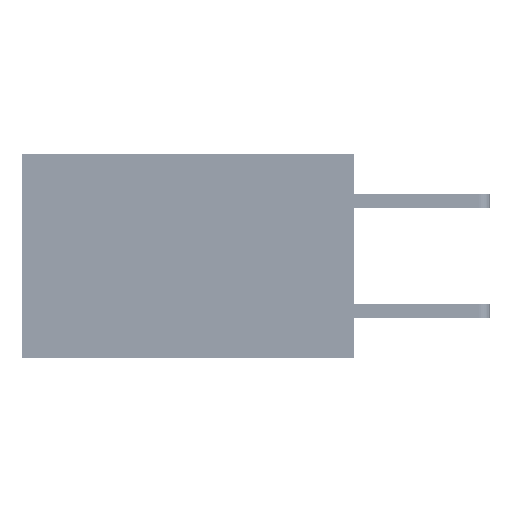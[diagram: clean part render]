
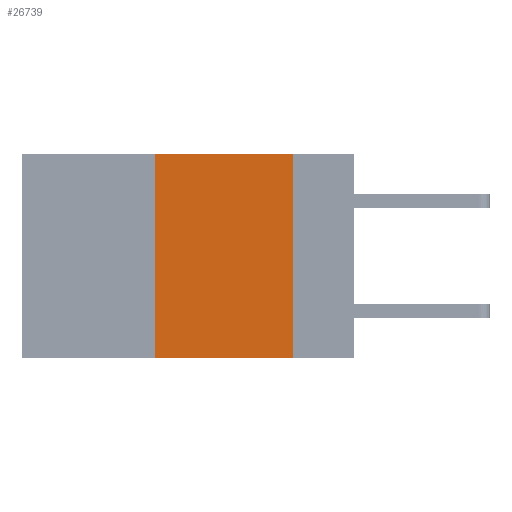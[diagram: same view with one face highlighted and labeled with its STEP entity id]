
A CAD part, left-side view. The second image highlights one B-rep face of the part: STEP entity #26739.
In plain terms, the highlighted planar face has unit normal (-1, 0, 0).
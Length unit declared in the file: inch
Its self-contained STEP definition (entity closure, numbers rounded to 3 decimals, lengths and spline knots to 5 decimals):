
#411 = VECTOR ( 'NONE', #22511, 39.37008 ) ;
#1099 = LINE ( 'NONE', #14853, #40923 ) ;
#1302 = CARTESIAN_POINT ( 'NONE',  ( 0., 0.11, 0. ) ) ;
#3840 = DIRECTION ( 'NONE',  ( 0., -1., 0. ) ) ;
#5320 = CARTESIAN_POINT ( 'NONE',  ( 0., 0.6, 0. ) ) ;
#7498 = CARTESIAN_POINT ( 'NONE',  ( 0., 0.6, 0. ) ) ;
#9156 = CARTESIAN_POINT ( 'NONE',  ( 0., 0.11, 0. ) ) ;
#10337 = VECTOR ( 'NONE', #22855, 39.37008 ) ;
#11505 = VECTOR ( 'NONE', #3840, 39.37008 ) ;
#14853 = CARTESIAN_POINT ( 'NONE',  ( 0., 0.6, -0.37 ) ) ;
#15875 = VERTEX_POINT ( 'NONE', #21773 ) ;
#17239 = AXIS2_PLACEMENT_3D ( 'NONE', #5320, #35069, #21687 ) ;
#17415 = CARTESIAN_POINT ( 'NONE',  ( 0., 0.36, 0. ) ) ;
#18458 = PLANE ( 'NONE',  #17239 ) ;
#20668 = EDGE_CURVE ( 'NONE', #32544, #28873, #37036, .T. ) ;
#20706 = CARTESIAN_POINT ( 'NONE',  ( 0., 0.11, -0.37 ) ) ;
#21687 = DIRECTION ( 'NONE',  ( 0., 0., -1. ) ) ;
#21773 = CARTESIAN_POINT ( 'NONE',  ( 0., 0.36, -0.37 ) ) ;
#22511 = DIRECTION ( 'NONE',  ( 0., 0., -1. ) ) ;
#22855 = DIRECTION ( 'NONE',  ( 0., 0., 1. ) ) ;
#25142 = FACE_OUTER_BOUND ( 'NONE', #33915, .T. ) ;
#26739 = ADVANCED_FACE ( 'NONE', ( #25142 ), #18458, .F. ) ;
#26741 = LINE ( 'NONE', #29549, #10337 ) ;
#28873 = VERTEX_POINT ( 'NONE', #1302 ) ;
#29549 = CARTESIAN_POINT ( 'NONE',  ( 0., 0.36, 0. ) ) ;
#30465 = ORIENTED_EDGE ( 'NONE', *, *, #36663, .F. ) ;
#32181 = EDGE_CURVE ( 'NONE', #15875, #35286, #1099, .T. ) ;
#32434 = ORIENTED_EDGE ( 'NONE', *, *, #32181, .T. ) ;
#32544 = VERTEX_POINT ( 'NONE', #17415 ) ;
#33915 = EDGE_LOOP ( 'NONE', ( #30465, #41339, #35921, #32434 ) ) ;
#35069 = DIRECTION ( 'NONE',  ( 1., 0., 0. ) ) ;
#35286 = VERTEX_POINT ( 'NONE', #20706 ) ;
#35921 = ORIENTED_EDGE ( 'NONE', *, *, #42275, .F. ) ;
#36663 = EDGE_CURVE ( 'NONE', #28873, #35286, #38694, .T. ) ;
#37036 = LINE ( 'NONE', #7498, #11505 ) ;
#38694 = LINE ( 'NONE', #9156, #411 ) ;
#40923 = VECTOR ( 'NONE', #41158, 39.37008 ) ;
#41158 = DIRECTION ( 'NONE',  ( 0., -1., 0. ) ) ;
#41339 = ORIENTED_EDGE ( 'NONE', *, *, #20668, .F. ) ;
#42275 = EDGE_CURVE ( 'NONE', #15875, #32544, #26741, .T. ) ;
